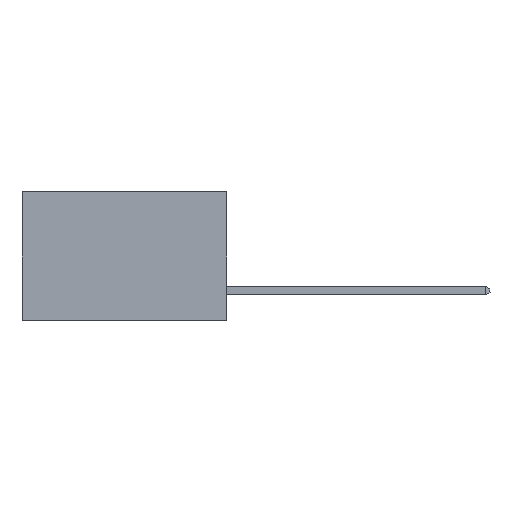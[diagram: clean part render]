
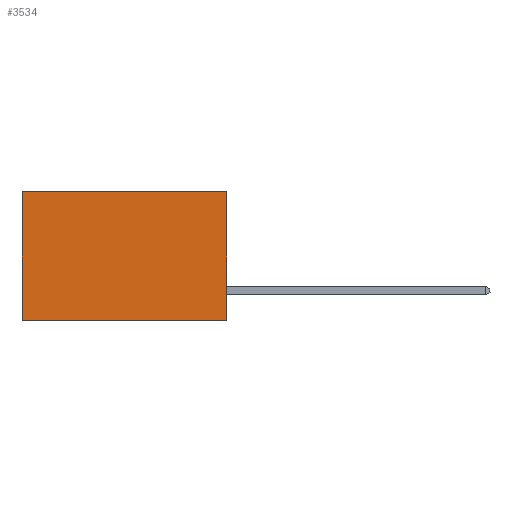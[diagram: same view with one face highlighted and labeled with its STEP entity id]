
A CAD part, left-side view. The second image highlights one B-rep face of the part: STEP entity #3534.
In plain terms, the highlighted planar face has unit normal (-1, 0, 0).
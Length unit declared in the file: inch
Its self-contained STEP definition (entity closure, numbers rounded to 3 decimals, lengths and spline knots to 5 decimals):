
#180 = EDGE_CURVE ( 'NONE', #11698, #2252, #1052, .T. ) ;
#386 = PLANE ( 'NONE',  #10227 ) ;
#570 = VERTEX_POINT ( 'NONE', #4940 ) ;
#1052 = LINE ( 'NONE', #9094, #3917 ) ;
#1204 = ORIENTED_EDGE ( 'NONE', *, *, #9773, .T. ) ;
#1222 = ORIENTED_EDGE ( 'NONE', *, *, #4567, .F. ) ;
#1319 = ORIENTED_EDGE ( 'NONE', *, *, #180, .F. ) ;
#1412 = LINE ( 'NONE', #13018, #11903 ) ;
#1429 = ORIENTED_EDGE ( 'NONE', *, *, #12204, .T. ) ;
#1912 = VERTEX_POINT ( 'NONE', #9341 ) ;
#1968 = CARTESIAN_POINT ( 'NONE',  ( 0.277, 0., -0.37 ) ) ;
#2150 = DIRECTION ( 'NONE',  ( 0., 1., 0. ) ) ;
#2252 = VERTEX_POINT ( 'NONE', #7808 ) ;
#2275 = CARTESIAN_POINT ( 'NONE',  ( 0.277, 0., 0. ) ) ;
#3249 = CARTESIAN_POINT ( 'NONE',  ( 0.277, 0.59, -0.37 ) ) ;
#3534 = ADVANCED_FACE ( 'NONE', ( #7710 ), #386, .F. ) ;
#3917 = VECTOR ( 'NONE', #10074, 39.37008 ) ;
#4567 = EDGE_CURVE ( 'NONE', #2252, #1912, #9382, .T. ) ;
#4674 = LINE ( 'NONE', #3249, #12893 ) ;
#4940 = CARTESIAN_POINT ( 'NONE',  ( 0.277, 0.59, 0. ) ) ;
#7209 = DIRECTION ( 'NONE',  ( 0., 1., 0. ) ) ;
#7710 = FACE_OUTER_BOUND ( 'NONE', #10552, .T. ) ;
#7808 = CARTESIAN_POINT ( 'NONE',  ( 0.277, 0., -0.37 ) ) ;
#9094 = CARTESIAN_POINT ( 'NONE',  ( 0.277, 0., -0.37 ) ) ;
#9341 = CARTESIAN_POINT ( 'NONE',  ( 0.277, 0.59, -0.37 ) ) ;
#9382 = LINE ( 'NONE', #1968, #11943 ) ;
#9773 = EDGE_CURVE ( 'NONE', #570, #1912, #4674, .T. ) ;
#10074 = DIRECTION ( 'NONE',  ( 0., 0., -1. ) ) ;
#10227 = AXIS2_PLACEMENT_3D ( 'NONE', #13215, #12567, #10297 ) ;
#10297 = DIRECTION ( 'NONE',  ( 0., 0., -1. ) ) ;
#10326 = DIRECTION ( 'NONE',  ( 0., 0., -1. ) ) ;
#10552 = EDGE_LOOP ( 'NONE', ( #1204, #1222, #1319, #1429 ) ) ;
#11698 = VERTEX_POINT ( 'NONE', #2275 ) ;
#11903 = VECTOR ( 'NONE', #7209, 39.37008 ) ;
#11943 = VECTOR ( 'NONE', #2150, 39.37008 ) ;
#12204 = EDGE_CURVE ( 'NONE', #11698, #570, #1412, .T. ) ;
#12567 = DIRECTION ( 'NONE',  ( 1., 0., 0. ) ) ;
#12893 = VECTOR ( 'NONE', #10326, 39.37008 ) ;
#13018 = CARTESIAN_POINT ( 'NONE',  ( 0.277, 0., 0. ) ) ;
#13215 = CARTESIAN_POINT ( 'NONE',  ( 0.277, 0., -0.37 ) ) ;
